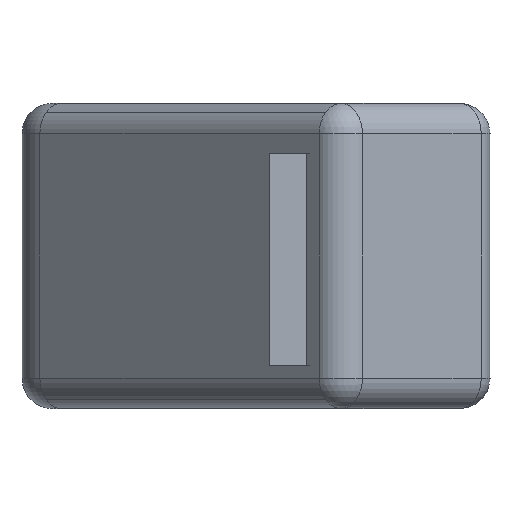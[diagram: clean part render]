
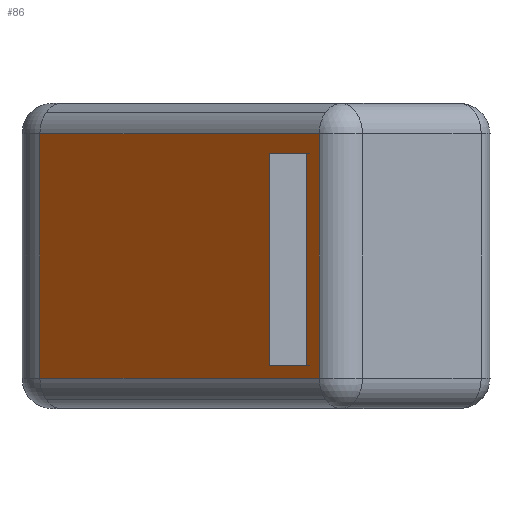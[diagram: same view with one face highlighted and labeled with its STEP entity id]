
A CAD part, front view. The second image highlights one B-rep face of the part: STEP entity #86.
In plain terms, the highlighted planar face has unit normal (-0.707, -0.707, 0).
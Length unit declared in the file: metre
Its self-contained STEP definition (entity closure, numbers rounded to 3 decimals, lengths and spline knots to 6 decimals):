
#86=ADVANCED_FACE('0:48',(#204,#205),#206,.T.);
#204=FACE_OUTER_BOUND('',#814,.T.);
#205=FACE_BOUND('',#815,.T.);
#206=PLANE('',#816);
#814=EDGE_LOOP('',(#1183,#1184,#1185,#1186));
#815=EDGE_LOOP('',(#1187,#1188,#1189,#1190));
#816=AXIS2_PLACEMENT_3D('',#1191,#1192,#1193);
#1183=ORIENTED_EDGE('',*,*,#1594,.F.);
#1184=ORIENTED_EDGE('',*,*,#1508,.F.);
#1185=ORIENTED_EDGE('',*,*,#1516,.F.);
#1186=ORIENTED_EDGE('',*,*,#1614,.T.);
#1187=ORIENTED_EDGE('',*,*,#1615,.F.);
#1188=ORIENTED_EDGE('',*,*,#1616,.F.);
#1189=ORIENTED_EDGE('',*,*,#1617,.F.);
#1190=ORIENTED_EDGE('',*,*,#1618,.F.);
#1191=CARTESIAN_POINT('',(0.020889,-0.056996,0.));
#1192=DIRECTION('',(-0.707,-0.707,-0.0));
#1193=DIRECTION('',(0.0,0.0,-1.0));
#1508=EDGE_CURVE('0:294',#1695,#1697,#1698,.T.);
#1516=EDGE_CURVE('0:297',#1711,#1695,#1713,.T.);
#1594=EDGE_CURVE('0:291',#1697,#1848,#1849,.T.);
#1614=EDGE_CURVE('0:252',#1711,#1848,#1872,.T.);
#1615=EDGE_CURVE('0:300',#1873,#1874,#1875,.T.);
#1616=EDGE_CURVE('0:303',#1876,#1873,#1877,.T.);
#1617=EDGE_CURVE('0:306',#1878,#1876,#1879,.T.);
#1618=EDGE_CURVE('0:309',#1874,#1878,#1880,.T.);
#1695=VERTEX_POINT('',#1986);
#1697=VERTEX_POINT('',#1988);
#1698=LINE('',#1989,#1990);
#1711=VERTEX_POINT('',#2006);
#1713=LINE('',#2008,#2009);
#1848=VERTEX_POINT('',#2185);
#1849=LINE('',#2186,#2187);
#1872=LINE('',#2215,#2216);
#1873=VERTEX_POINT('',#2217);
#1874=VERTEX_POINT('',#2218);
#1875=LINE('',#2219,#2220);
#1876=VERTEX_POINT('',#2221);
#1877=LINE('',#2222,#2223);
#1878=VERTEX_POINT('',#2224);
#1879=LINE('',#2225,#2226);
#1880=LINE('',#2227,#2228);
#1986=CARTESIAN_POINT('',(0.001172,-0.037278,0.002));
#1988=CARTESIAN_POINT('',(0.001172,-0.037278,0.018));
#1989=CARTESIAN_POINT('',(0.001172,-0.037278,0.));
#1990=VECTOR('',#2368,1.0);
#2006=CARTESIAN_POINT('',(0.019475,-0.055581,0.002));
#2008=CARTESIAN_POINT('',(0.003696,-0.039803,0.002));
#2009=VECTOR('',#2384,1.0);
#2185=CARTESIAN_POINT('',(0.019475,-0.055581,0.018));
#2186=CARTESIAN_POINT('',(0.003696,-0.039803,0.018));
#2187=VECTOR('',#2534,1.0);
#2215=CARTESIAN_POINT('',(0.019475,-0.055581,0.));
#2216=VECTOR('',#2582,0.001);
#2217=CARTESIAN_POINT('',(0.018622,-0.054728,0.016734));
#2218=CARTESIAN_POINT('',(0.016216,-0.052323,0.016734));
#2219=CARTESIAN_POINT('',(0.018622,-0.054728,0.016734));
#2220=VECTOR('',#2583,0.001);
#2221=CARTESIAN_POINT('',(0.018622,-0.054728,0.002818));
#2222=CARTESIAN_POINT('',(0.018622,-0.054728,0.002818));
#2223=VECTOR('',#2584,0.001);
#2224=CARTESIAN_POINT('',(0.016216,-0.052323,0.002818));
#2225=CARTESIAN_POINT('',(0.016216,-0.052323,0.002818));
#2226=VECTOR('',#2585,0.001);
#2227=CARTESIAN_POINT('',(0.016216,-0.052323,0.016734));
#2228=VECTOR('',#2586,0.001);
#2368=DIRECTION('',(0.0,0.0,1.0));
#2384=DIRECTION('',(-0.707,0.707,0.0));
#2534=DIRECTION('',(0.707,-0.707,-0.0));
#2582=DIRECTION('',(0.0,0.0,1.0));
#2583=DIRECTION('',(-0.707,0.707,0.0));
#2584=DIRECTION('',(0.0,0.0,1.0));
#2585=DIRECTION('',(0.707,-0.707,0.0));
#2586=DIRECTION('',(0.0,0.0,-1.0));
